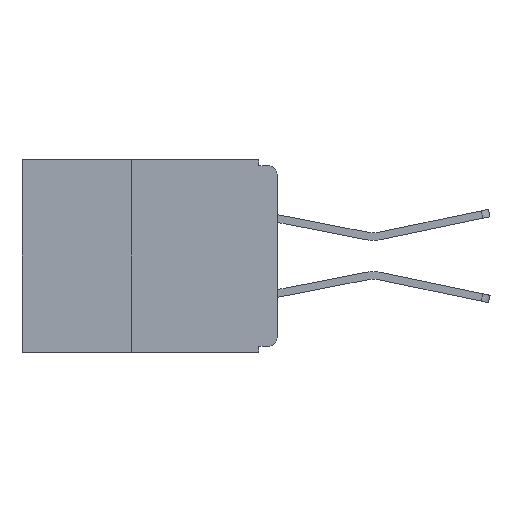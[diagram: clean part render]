
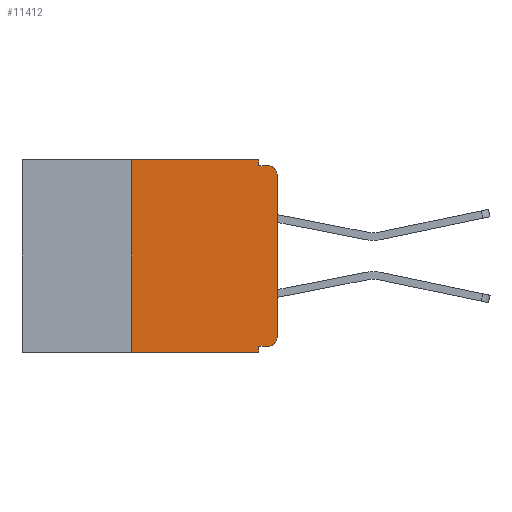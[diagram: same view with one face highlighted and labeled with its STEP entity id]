
A CAD part, left-side view. The second image highlights one B-rep face of the part: STEP entity #11412.
In plain terms, the highlighted planar face has unit normal (-1, 0, 0).
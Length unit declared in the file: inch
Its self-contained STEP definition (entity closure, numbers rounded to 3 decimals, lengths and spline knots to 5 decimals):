
#17 = VERTEX_POINT ( 'NONE', #13718 ) ;
#155 = LINE ( 'NONE', #9832, #9251 ) ;
#903 = EDGE_LOOP ( 'NONE', ( #7285, #13326, #7997, #5292, #8688, #11742, #7644, #4969, #13816, #14131 ) ) ;
#1095 = CIRCLE ( 'NONE', #9921, 0.015 ) ;
#1307 = LINE ( 'NONE', #2589, #13085 ) ;
#1751 = CARTESIAN_POINT ( 'NONE',  ( 0., 0.031, -0.33 ) ) ;
#2102 = VERTEX_POINT ( 'NONE', #2180 ) ;
#2180 = CARTESIAN_POINT ( 'NONE',  ( 0., 0.015, -0.01 ) ) ;
#2185 = VECTOR ( 'NONE', #9981, 39.37008 ) ;
#2419 = VECTOR ( 'NONE', #13061, 39.37008 ) ;
#2589 = CARTESIAN_POINT ( 'NONE',  ( 0., 0., 0. ) ) ;
#2620 = DIRECTION ( 'NONE',  ( -1., 0., 0. ) ) ;
#3107 = EDGE_CURVE ( 'NONE', #8179, #8448, #155, .T. ) ;
#3395 = LINE ( 'NONE', #5069, #11927 ) ;
#3472 = CARTESIAN_POINT ( 'NONE',  ( 0., 0.25, -0.33 ) ) ;
#4492 = EDGE_CURVE ( 'NONE', #9970, #10968, #3395, .T. ) ;
#4611 = DIRECTION ( 'NONE',  ( 0., 0., 1. ) ) ;
#4631 = LINE ( 'NONE', #3472, #10249 ) ;
#4812 = CARTESIAN_POINT ( 'NONE',  ( 0., 0.015, -0.32 ) ) ;
#4828 = DIRECTION ( 'NONE',  ( 0., -1., 0. ) ) ;
#4829 = LINE ( 'NONE', #14150, #2185 ) ;
#4969 = ORIENTED_EDGE ( 'NONE', *, *, #9856, .F. ) ;
#5069 = CARTESIAN_POINT ( 'NONE',  ( 0., 0.437, -0.33 ) ) ;
#5178 = VERTEX_POINT ( 'NONE', #13946 ) ;
#5292 = ORIENTED_EDGE ( 'NONE', *, *, #12616, .F. ) ;
#5573 = VERTEX_POINT ( 'NONE', #10602 ) ;
#5592 = EDGE_CURVE ( 'NONE', #7479, #2102, #12361, .T. ) ;
#5682 = EDGE_CURVE ( 'NONE', #8179, #17, #13830, .T. ) ;
#5936 = DIRECTION ( 'NONE',  ( 0., 0., 1. ) ) ;
#5983 = DIRECTION ( 'NONE',  ( 1., 0., 0. ) ) ;
#6087 = CARTESIAN_POINT ( 'NONE',  ( 0., 0.031, -0.01 ) ) ;
#7219 = CARTESIAN_POINT ( 'NONE',  ( 0., 0.031, 0. ) ) ;
#7285 = ORIENTED_EDGE ( 'NONE', *, *, #8835, .T. ) ;
#7479 = VERTEX_POINT ( 'NONE', #6087 ) ;
#7601 = CARTESIAN_POINT ( 'NONE',  ( 0., 0.031, -0.32 ) ) ;
#7644 = ORIENTED_EDGE ( 'NONE', *, *, #4492, .T. ) ;
#7724 = CARTESIAN_POINT ( 'NONE',  ( 0., 0.437, 0. ) ) ;
#7905 = EDGE_CURVE ( 'NONE', #11419, #5573, #11686, .T. ) ;
#7997 = ORIENTED_EDGE ( 'NONE', *, *, #5592, .F. ) ;
#8179 = VERTEX_POINT ( 'NONE', #4812 ) ;
#8256 = PLANE ( 'NONE',  #10889 ) ;
#8300 = CARTESIAN_POINT ( 'NONE',  ( 0., 0.25, 0. ) ) ;
#8448 = VERTEX_POINT ( 'NONE', #7601 ) ;
#8688 = ORIENTED_EDGE ( 'NONE', *, *, #7905, .F. ) ;
#8835 = EDGE_CURVE ( 'NONE', #17, #5178, #1307, .T. ) ;
#9251 = VECTOR ( 'NONE', #9712, 39.37008 ) ;
#9299 = DIRECTION ( 'NONE',  ( 0., 0., -1. ) ) ;
#9303 = DIRECTION ( 'NONE',  ( -1., 0., 0. ) ) ;
#9317 = CARTESIAN_POINT ( 'NONE',  ( 0., 0.015, -0.305 ) ) ;
#9375 = CARTESIAN_POINT ( 'NONE',  ( 0., 0.015, -0.025 ) ) ;
#9466 = EDGE_CURVE ( 'NONE', #5178, #2102, #1095, .T. ) ;
#9712 = DIRECTION ( 'NONE',  ( 0., 1., 0. ) ) ;
#9832 = CARTESIAN_POINT ( 'NONE',  ( 0., 0., -0.32 ) ) ;
#9856 = EDGE_CURVE ( 'NONE', #8448, #10968, #4829, .T. ) ;
#9921 = AXIS2_PLACEMENT_3D ( 'NONE', #9375, #2620, #10465 ) ;
#9970 = VERTEX_POINT ( 'NONE', #12285 ) ;
#9981 = DIRECTION ( 'NONE',  ( 0., 0., -1. ) ) ;
#10011 = DIRECTION ( 'NONE',  ( 0., -1., 0. ) ) ;
#10064 = CARTESIAN_POINT ( 'NONE',  ( 0., 0., -0.01 ) ) ;
#10249 = VECTOR ( 'NONE', #4611, 39.37008 ) ;
#10418 = FACE_OUTER_BOUND ( 'NONE', #903, .T. ) ;
#10432 = CARTESIAN_POINT ( 'NONE',  ( 0., 0.437, 0. ) ) ;
#10465 = DIRECTION ( 'NONE',  ( 0., 0., -1. ) ) ;
#10503 = EDGE_CURVE ( 'NONE', #9970, #11419, #4631, .T. ) ;
#10519 = AXIS2_PLACEMENT_3D ( 'NONE', #9317, #9303, #9299 ) ;
#10602 = CARTESIAN_POINT ( 'NONE',  ( 0., 0.031, 0. ) ) ;
#10714 = VECTOR ( 'NONE', #13644, 39.37008 ) ;
#10889 = AXIS2_PLACEMENT_3D ( 'NONE', #10432, #5983, #13582 ) ;
#10968 = VERTEX_POINT ( 'NONE', #1751 ) ;
#11412 = ADVANCED_FACE ( 'NONE', ( #10418 ), #8256, .F. ) ;
#11419 = VERTEX_POINT ( 'NONE', #8300 ) ;
#11686 = LINE ( 'NONE', #7724, #2419 ) ;
#11742 = ORIENTED_EDGE ( 'NONE', *, *, #10503, .F. ) ;
#11927 = VECTOR ( 'NONE', #4828, 39.37008 ) ;
#12049 = VECTOR ( 'NONE', #10011, 39.37008 ) ;
#12285 = CARTESIAN_POINT ( 'NONE',  ( 0., 0.25, -0.33 ) ) ;
#12361 = LINE ( 'NONE', #10064, #12049 ) ;
#12616 = EDGE_CURVE ( 'NONE', #5573, #7479, #13487, .T. ) ;
#13061 = DIRECTION ( 'NONE',  ( 0., -1., 0. ) ) ;
#13085 = VECTOR ( 'NONE', #5936, 39.37008 ) ;
#13326 = ORIENTED_EDGE ( 'NONE', *, *, #9466, .T. ) ;
#13487 = LINE ( 'NONE', #7219, #10714 ) ;
#13582 = DIRECTION ( 'NONE',  ( 0., 0., -1. ) ) ;
#13644 = DIRECTION ( 'NONE',  ( 0., 0., -1. ) ) ;
#13718 = CARTESIAN_POINT ( 'NONE',  ( 0., 0., -0.305 ) ) ;
#13816 = ORIENTED_EDGE ( 'NONE', *, *, #3107, .F. ) ;
#13830 = CIRCLE ( 'NONE', #10519, 0.015 ) ;
#13946 = CARTESIAN_POINT ( 'NONE',  ( 0., 0., -0.025 ) ) ;
#14131 = ORIENTED_EDGE ( 'NONE', *, *, #5682, .T. ) ;
#14150 = CARTESIAN_POINT ( 'NONE',  ( 0., 0.031, -0.33 ) ) ;
